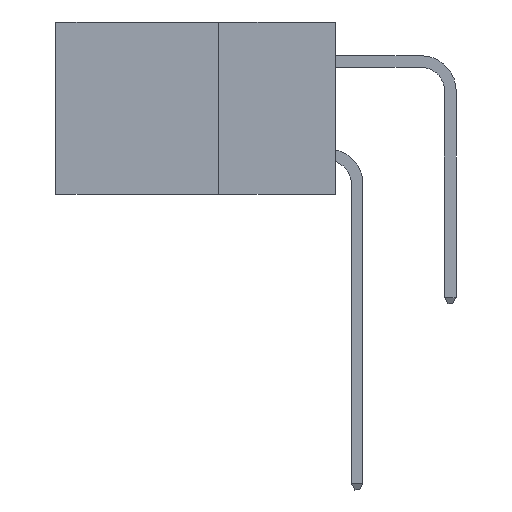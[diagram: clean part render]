
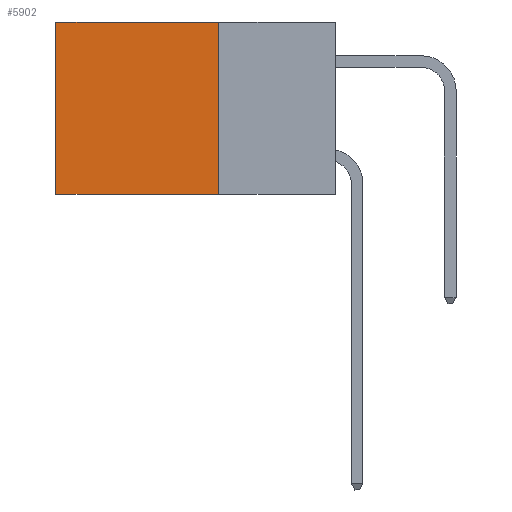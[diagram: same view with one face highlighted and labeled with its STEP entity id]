
A CAD part, left-side view. The second image highlights one B-rep face of the part: STEP entity #5902.
In plain terms, the highlighted planar face has unit normal (-1, 0, 0).
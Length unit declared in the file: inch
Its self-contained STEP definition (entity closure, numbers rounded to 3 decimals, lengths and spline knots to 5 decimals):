
#606 = CARTESIAN_POINT ( 'NONE',  ( 0.2875, 0.25, 0. ) ) ;
#1534 = FACE_OUTER_BOUND ( 'NONE', #5440, .T. ) ;
#3501 = DIRECTION ( 'NONE',  ( 0., 0., -1. ) ) ;
#4976 = VECTOR ( 'NONE', #12209, 39.37008 ) ;
#5274 = DIRECTION ( 'NONE',  ( 0., 0., -1. ) ) ;
#5440 = EDGE_LOOP ( 'NONE', ( #26312, #13031, #15034, #12293 ) ) ;
#5670 = EDGE_CURVE ( 'NONE', #20883, #10266, #26477, .T. ) ;
#5902 = ADVANCED_FACE ( 'NONE', ( #1534 ), #10234, .F. ) ;
#8562 = CARTESIAN_POINT ( 'NONE',  ( 0.2875, 0.6, 0. ) ) ;
#9879 = EDGE_CURVE ( 'NONE', #17909, #20883, #23022, .T. ) ;
#9895 = VECTOR ( 'NONE', #23099, 39.37008 ) ;
#10234 = PLANE ( 'NONE',  #21176 ) ;
#10266 = VERTEX_POINT ( 'NONE', #24407 ) ;
#10505 = EDGE_CURVE ( 'NONE', #27510, #10266, #22632, .T. ) ;
#11288 = VECTOR ( 'NONE', #5274, 39.37008 ) ;
#12124 = CARTESIAN_POINT ( 'NONE',  ( 0.2875, 0.6, 0. ) ) ;
#12209 = DIRECTION ( 'NONE',  ( 0., 1., 0. ) ) ;
#12293 = ORIENTED_EDGE ( 'NONE', *, *, #9879, .T. ) ;
#13031 = ORIENTED_EDGE ( 'NONE', *, *, #10505, .F. ) ;
#13706 = VECTOR ( 'NONE', #22064, 39.37008 ) ;
#13914 = CARTESIAN_POINT ( 'NONE',  ( 0.2875, 0.25, 0. ) ) ;
#14832 = DIRECTION ( 'NONE',  ( 1., 0., 0. ) ) ;
#15034 = ORIENTED_EDGE ( 'NONE', *, *, #25861, .F. ) ;
#17909 = VERTEX_POINT ( 'NONE', #606 ) ;
#18039 = CARTESIAN_POINT ( 'NONE',  ( 0.2875, 0.25, -0.37 ) ) ;
#20883 = VERTEX_POINT ( 'NONE', #8562 ) ;
#21176 = AXIS2_PLACEMENT_3D ( 'NONE', #28085, #14832, #3501 ) ;
#22064 = DIRECTION ( 'NONE',  ( 0., 0., -1. ) ) ;
#22632 = LINE ( 'NONE', #23159, #4976 ) ;
#23022 = LINE ( 'NONE', #13914, #9895 ) ;
#23099 = DIRECTION ( 'NONE',  ( 0., 1., 0. ) ) ;
#23159 = CARTESIAN_POINT ( 'NONE',  ( 0.2875, 0.25, -0.37 ) ) ;
#24407 = CARTESIAN_POINT ( 'NONE',  ( 0.2875, 0.6, -0.37 ) ) ;
#24424 = LINE ( 'NONE', #26777, #13706 ) ;
#25861 = EDGE_CURVE ( 'NONE', #17909, #27510, #24424, .T. ) ;
#26312 = ORIENTED_EDGE ( 'NONE', *, *, #5670, .T. ) ;
#26477 = LINE ( 'NONE', #12124, #11288 ) ;
#26777 = CARTESIAN_POINT ( 'NONE',  ( 0.2875, 0.25, 0. ) ) ;
#27510 = VERTEX_POINT ( 'NONE', #18039 ) ;
#28085 = CARTESIAN_POINT ( 'NONE',  ( 0.2875, 0.25, 0. ) ) ;
